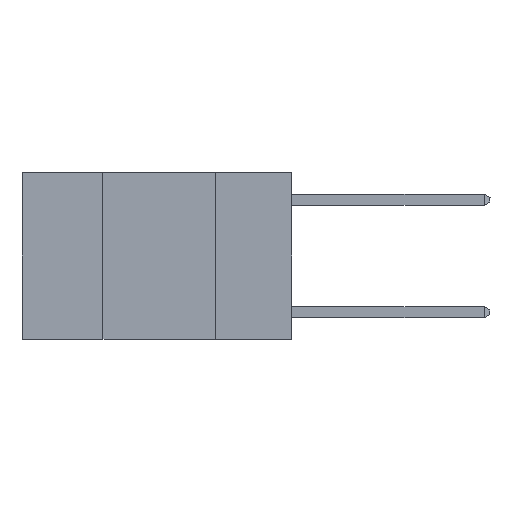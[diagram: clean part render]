
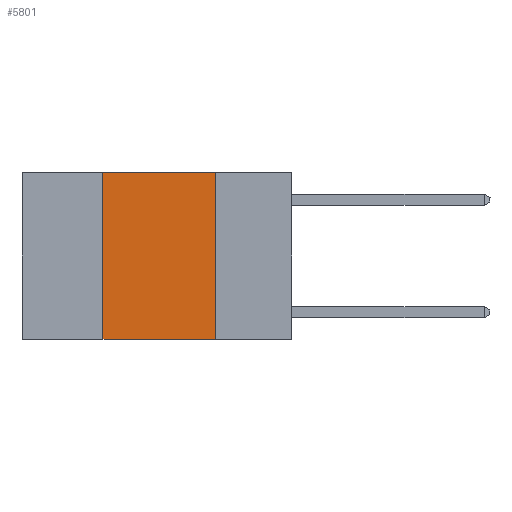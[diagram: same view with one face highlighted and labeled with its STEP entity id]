
A CAD part, left-side view. The second image highlights one B-rep face of the part: STEP entity #5801.
In plain terms, the highlighted planar face has unit normal (-1, 0, 0).
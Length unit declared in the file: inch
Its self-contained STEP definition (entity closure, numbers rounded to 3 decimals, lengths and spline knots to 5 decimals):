
#268 = DIRECTION ( 'NONE',  ( 0., 0., -1. ) ) ;
#478 = VECTOR ( 'NONE', #11427, 39.37008 ) ;
#798 = CARTESIAN_POINT ( 'NONE',  ( 0., 0.42, -0.37 ) ) ;
#886 = CARTESIAN_POINT ( 'NONE',  ( 0., 0.6, -0.37 ) ) ;
#1281 = ORIENTED_EDGE ( 'NONE', *, *, #5962, .F. ) ;
#3055 = EDGE_CURVE ( 'NONE', #6331, #9402, #6214, .T. ) ;
#3279 = CARTESIAN_POINT ( 'NONE',  ( 0., 0.42, 0. ) ) ;
#3699 = ORIENTED_EDGE ( 'NONE', *, *, #3055, .F. ) ;
#4598 = LINE ( 'NONE', #886, #478 ) ;
#5801 = ADVANCED_FACE ( 'NONE', ( #11701 ), #6044, .F. ) ;
#5962 = EDGE_CURVE ( 'NONE', #14031, #6331, #11169, .T. ) ;
#6044 = PLANE ( 'NONE',  #8469 ) ;
#6214 = LINE ( 'NONE', #8510, #6682 ) ;
#6331 = VERTEX_POINT ( 'NONE', #13297 ) ;
#6682 = VECTOR ( 'NONE', #268, 39.37008 ) ;
#8134 = EDGE_CURVE ( 'NONE', #8466, #14031, #13797, .T. ) ;
#8257 = CARTESIAN_POINT ( 'NONE',  ( 0., 0.6, 0. ) ) ;
#8466 = VERTEX_POINT ( 'NONE', #798 ) ;
#8469 = AXIS2_PLACEMENT_3D ( 'NONE', #8257, #10779, #9626 ) ;
#8510 = CARTESIAN_POINT ( 'NONE',  ( 0., 0.17, 0. ) ) ;
#8655 = CARTESIAN_POINT ( 'NONE',  ( 0., 0.6, 0. ) ) ;
#9402 = VERTEX_POINT ( 'NONE', #12135 ) ;
#9626 = DIRECTION ( 'NONE',  ( 0., 0., -1. ) ) ;
#10333 = CARTESIAN_POINT ( 'NONE',  ( 0., 0.42, 0. ) ) ;
#10779 = DIRECTION ( 'NONE',  ( 1., 0., 0. ) ) ;
#10878 = ORIENTED_EDGE ( 'NONE', *, *, #8134, .F. ) ;
#10883 = ORIENTED_EDGE ( 'NONE', *, *, #12078, .T. ) ;
#11169 = LINE ( 'NONE', #8655, #13363 ) ;
#11279 = EDGE_LOOP ( 'NONE', ( #3699, #1281, #10878, #10883 ) ) ;
#11427 = DIRECTION ( 'NONE',  ( 0., -1., 0. ) ) ;
#11495 = DIRECTION ( 'NONE',  ( 0., 0., 1. ) ) ;
#11701 = FACE_OUTER_BOUND ( 'NONE', #11279, .T. ) ;
#12002 = DIRECTION ( 'NONE',  ( 0., -1., 0. ) ) ;
#12078 = EDGE_CURVE ( 'NONE', #8466, #9402, #4598, .T. ) ;
#12135 = CARTESIAN_POINT ( 'NONE',  ( 0., 0.17, -0.37 ) ) ;
#12545 = VECTOR ( 'NONE', #11495, 39.37008 ) ;
#13297 = CARTESIAN_POINT ( 'NONE',  ( 0., 0.17, 0. ) ) ;
#13363 = VECTOR ( 'NONE', #12002, 39.37008 ) ;
#13797 = LINE ( 'NONE', #3279, #12545 ) ;
#14031 = VERTEX_POINT ( 'NONE', #10333 ) ;
